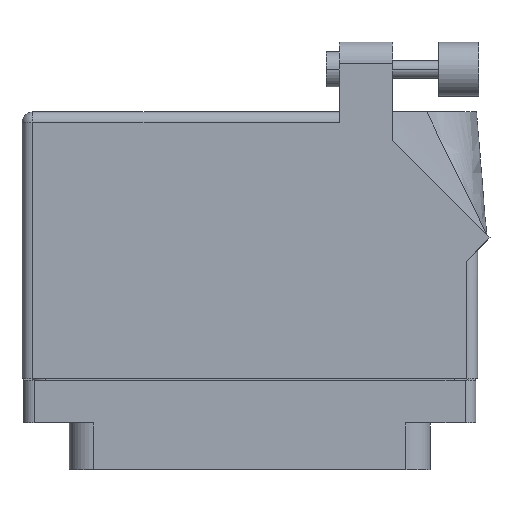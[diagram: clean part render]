
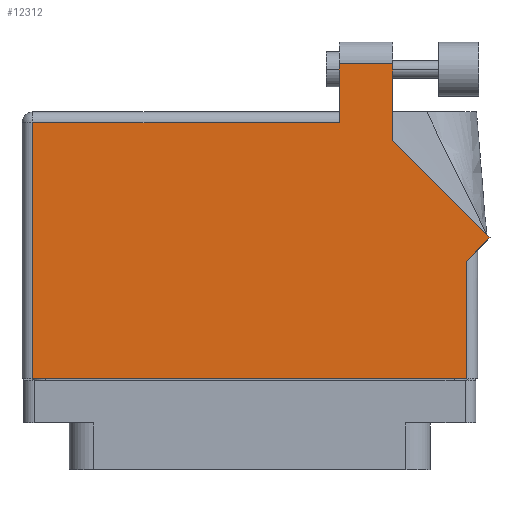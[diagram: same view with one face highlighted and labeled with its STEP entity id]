
A CAD part, front view. The second image highlights one B-rep face of the part: STEP entity #12312.
In plain terms, the highlighted face is planar.
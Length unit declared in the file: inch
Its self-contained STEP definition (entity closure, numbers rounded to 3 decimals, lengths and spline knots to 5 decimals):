
#20 = VERTEX_POINT ( 'NONE', #19298 ) ;
#1077 = CARTESIAN_POINT ( 'NONE',  ( 0.513, 1.705, 0.455 ) ) ;
#1467 = CARTESIAN_POINT ( 'NONE',  ( 1.306, 0.637, 0.455 ) ) ;
#2536 = LINE ( 'NONE', #19757, #32048 ) ;
#2656 = EDGE_CURVE ( 'NONE', #44966, #20, #44775, .T. ) ;
#2859 = ORIENTED_EDGE ( 'NONE', *, *, #33031, .T. ) ;
#2998 = ORIENTED_EDGE ( 'NONE', *, *, #2656, .T. ) ;
#3601 = EDGE_CURVE ( 'NONE', #6408, #46270, #30852, .T. ) ;
#4449 = DIRECTION ( 'NONE',  ( 0., 1., 0. ) ) ;
#5319 = EDGE_CURVE ( 'NONE', #20, #35679, #24263, .T. ) ;
#6387 = DIRECTION ( 'NONE',  ( 0., -1., 0. ) ) ;
#6408 = VERTEX_POINT ( 'NONE', #1077 ) ;
#9275 = AXIS2_PLACEMENT_3D ( 'NONE', #13783, #21809, #37220 ) ;
#9567 = CARTESIAN_POINT ( 'NONE',  ( 0.82, 1.26442, 0.455 ) ) ;
#9659 = FACE_OUTER_BOUND ( 'NONE', #16411, .T. ) ;
#9868 = CARTESIAN_POINT ( 'NONE',  ( 0.82, 1.705, 0.455 ) ) ;
#11067 = ORIENTED_EDGE ( 'NONE', *, *, #3601, .T. ) ;
#11904 = DIRECTION ( 'NONE',  ( -1., 0., 0. ) ) ;
#12312 = ADVANCED_FACE ( 'NONE', ( #9659 ), #33198, .F. ) ;
#12555 = CARTESIAN_POINT ( 'NONE',  ( 1.244, 0.637, 0.455 ) ) ;
#12689 = VECTOR ( 'NONE', #43314, 39.37008 ) ;
#13065 = CARTESIAN_POINT ( 'NONE',  ( 1.244, 0.575, 0.455 ) ) ;
#13589 = EDGE_CURVE ( 'NONE', #37985, #30494, #33951, .T. ) ;
#13783 = CARTESIAN_POINT ( 'NONE',  ( -1.306, 1.43, 0.455 ) ) ;
#13989 = DIRECTION ( 'NONE',  ( 0.707, 0.707, 0. ) ) ;
#14448 = VECTOR ( 'NONE', #4449, 39.37008 ) ;
#15635 = CARTESIAN_POINT ( 'NONE',  ( 0.513, 1.43, 0.455 ) ) ;
#16411 = EDGE_LOOP ( 'NONE', ( #38725, #2859, #11067, #25683, #2998, #17721, #18490, #48510, #18106 ) ) ;
#17063 = DIRECTION ( 'NONE',  ( 1., 0., 0. ) ) ;
#17388 = VECTOR ( 'NONE', #17063, 39.37008 ) ;
#17721 = ORIENTED_EDGE ( 'NONE', *, *, #5319, .T. ) ;
#18106 = ORIENTED_EDGE ( 'NONE', *, *, #13589, .T. ) ;
#18490 = ORIENTED_EDGE ( 'NONE', *, *, #33590, .T. ) ;
#19298 = CARTESIAN_POINT ( 'NONE',  ( -1.244, -0.1, 0.455 ) ) ;
#19757 = CARTESIAN_POINT ( 'NONE',  ( 0.513, 1.705, 0.455 ) ) ;
#20727 = LINE ( 'NONE', #27580, #21970 ) ;
#20740 = CARTESIAN_POINT ( 'NONE',  ( 1.244, -0.1, 0.455 ) ) ;
#21232 = DIRECTION ( 'NONE',  ( -0.707, 0.707, 0. ) ) ;
#21809 = DIRECTION ( 'NONE',  ( 0., 0., -1. ) ) ;
#21970 = VECTOR ( 'NONE', #51713, 39.37008 ) ;
#22972 = CARTESIAN_POINT ( 'NONE',  ( 0.513, 1.368, 0.455 ) ) ;
#23690 = CARTESIAN_POINT ( 'NONE',  ( -1.306, -0.1, 0.455 ) ) ;
#24263 = LINE ( 'NONE', #23690, #17388 ) ;
#25216 = LINE ( 'NONE', #1467, #42774 ) ;
#25683 = ORIENTED_EDGE ( 'NONE', *, *, #36465, .T. ) ;
#25795 = CARTESIAN_POINT ( 'NONE',  ( 1.37671, 0.70771, 0.455 ) ) ;
#27580 = CARTESIAN_POINT ( 'NONE',  ( -1.306, 1.368, 0.455 ) ) ;
#28126 = VERTEX_POINT ( 'NONE', #9868 ) ;
#30494 = VERTEX_POINT ( 'NONE', #9567 ) ;
#30852 = LINE ( 'NONE', #15635, #12689 ) ;
#32048 = VECTOR ( 'NONE', #11904, 39.37008 ) ;
#33031 = EDGE_CURVE ( 'NONE', #28126, #6408, #2536, .T. ) ;
#33198 = PLANE ( 'NONE',  #9275 ) ;
#33295 = VECTOR ( 'NONE', #21232, 39.37008 ) ;
#33556 = VERTEX_POINT ( 'NONE', #13065 ) ;
#33590 = EDGE_CURVE ( 'NONE', #35679, #33556, #38224, .T. ) ;
#33951 = LINE ( 'NONE', #25795, #33295 ) ;
#34109 = VECTOR ( 'NONE', #6387, 39.37008 ) ;
#35679 = VERTEX_POINT ( 'NONE', #20740 ) ;
#36465 = EDGE_CURVE ( 'NONE', #46270, #44966, #20727, .T. ) ;
#37220 = DIRECTION ( 'NONE',  ( -1., 0., 0. ) ) ;
#37985 = VERTEX_POINT ( 'NONE', #40913 ) ;
#38224 = LINE ( 'NONE', #12555, #14448 ) ;
#38298 = CARTESIAN_POINT ( 'NONE',  ( -1.244, 1.368, 0.455 ) ) ;
#38665 = DIRECTION ( 'NONE',  ( 0., 1., 0. ) ) ;
#38725 = ORIENTED_EDGE ( 'NONE', *, *, #51022, .T. ) ;
#40913 = CARTESIAN_POINT ( 'NONE',  ( 1.37671, 0.70771, 0.455 ) ) ;
#42250 = CARTESIAN_POINT ( 'NONE',  ( 0.82, 1.26442, 0.455 ) ) ;
#42774 = VECTOR ( 'NONE', #13989, 39.37008 ) ;
#43314 = DIRECTION ( 'NONE',  ( 0., -1., 0. ) ) ;
#44775 = LINE ( 'NONE', #50159, #34109 ) ;
#44966 = VERTEX_POINT ( 'NONE', #38298 ) ;
#46270 = VERTEX_POINT ( 'NONE', #22972 ) ;
#46968 = VECTOR ( 'NONE', #38665, 39.37008 ) ;
#47931 = EDGE_CURVE ( 'NONE', #33556, #37985, #25216, .T. ) ;
#48510 = ORIENTED_EDGE ( 'NONE', *, *, #47931, .T. ) ;
#49451 = LINE ( 'NONE', #42250, #46968 ) ;
#50159 = CARTESIAN_POINT ( 'NONE',  ( -1.244, -0.1, 0.455 ) ) ;
#51022 = EDGE_CURVE ( 'NONE', #30494, #28126, #49451, .T. ) ;
#51713 = DIRECTION ( 'NONE',  ( -1., 0., 0. ) ) ;
